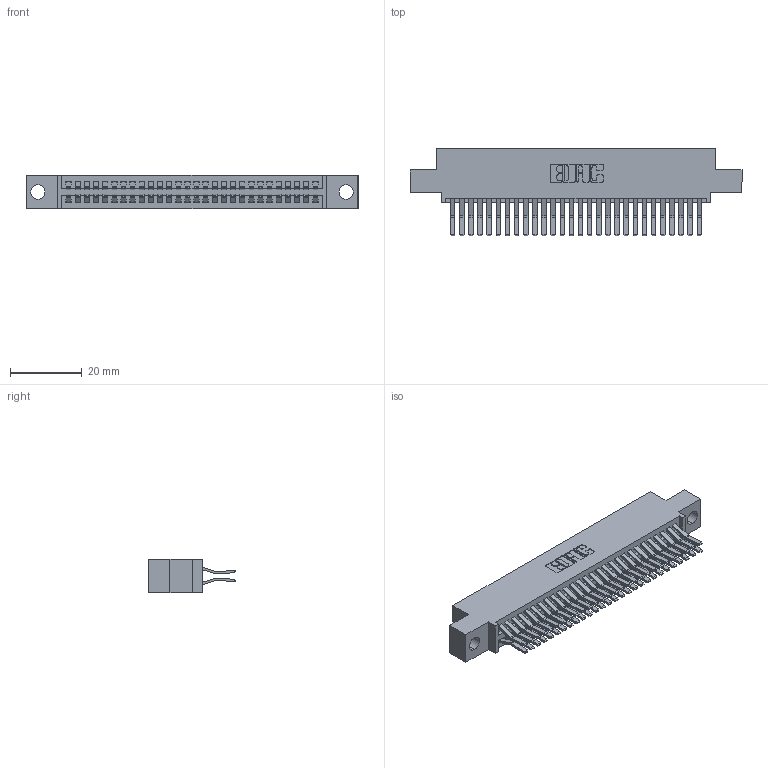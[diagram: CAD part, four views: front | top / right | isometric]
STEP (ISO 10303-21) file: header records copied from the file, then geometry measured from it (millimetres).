
FILE_DESCRIPTION (( 'STEP AP203' ), '1' );
FILE_NAME ('345-056-560-504.STEP', '2021-05-20T04:52:15', ( '' ), ( '' ), 'SwSTEP 2.0', 'SolidWorks 2020', '' );
FILE_SCHEMA (( 'CONFIG_CONTROL_DESIGN' ));
Length unit declared in the file: inch
Products named in the file (3): 345 Part_0.110 Offset - 0.156 Dia-TI; 345-056-560-504; 345-292-001_560 Tail
Assembly tree (57 placements, depth 2):
  345-056-560-504
    345 Part_0.110 Offset - 0.156 Dia-TI
    345-292-001_560 Tail  x56
Bounding box: 92.33 x 24.45 x 9.4 mm (x, y, z)
Volume: 9026.7 mm3; surface area: 13960.3 mm2
Topology: 57 solids, 57 shells, 3056 faces, 9069 edges, 5970 vertices
Faces by surface type: plane 1946, cylinder 1110
Entity records: 24493 total; most frequent: CARTESIAN_POINT 4126, ORIENTED_EDGE 4058, DIRECTION 3657, EDGE_CURVE 2029, VECTOR 1781, LINE 1781, VERTEX_POINT 1350, AXIS2_PLACEMENT_3D 938
